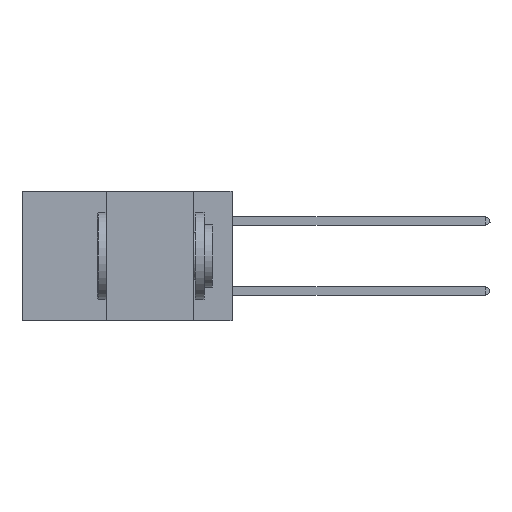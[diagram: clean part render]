
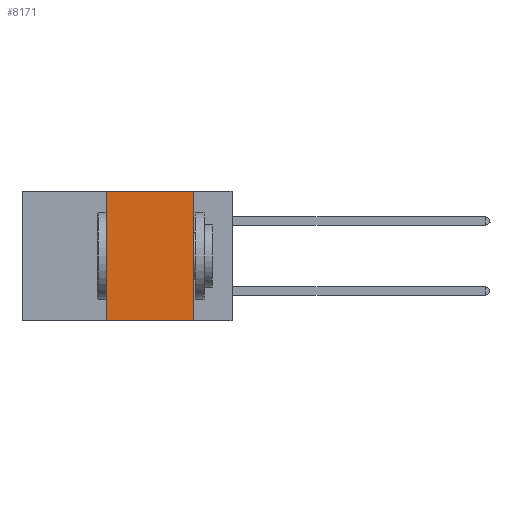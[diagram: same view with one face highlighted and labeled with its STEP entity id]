
A CAD part, left-side view. The second image highlights one B-rep face of the part: STEP entity #8171.
In plain terms, the highlighted planar face has unit normal (-1, 0, 0).
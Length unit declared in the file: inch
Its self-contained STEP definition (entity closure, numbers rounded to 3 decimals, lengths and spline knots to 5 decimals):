
#1097 = CARTESIAN_POINT ( 'NONE',  ( 0., 0.6, -0.37 ) ) ;
#3620 = FACE_OUTER_BOUND ( 'NONE', #18845, .T. ) ;
#3628 = LINE ( 'NONE', #43372, #38370 ) ;
#4054 = ORIENTED_EDGE ( 'NONE', *, *, #33703, .F. ) ;
#4055 = CARTESIAN_POINT ( 'NONE',  ( 0., 0.36, -0.37 ) ) ;
#6452 = DIRECTION ( 'NONE',  ( 0., -1., 0. ) ) ;
#7002 = LINE ( 'NONE', #9540, #31798 ) ;
#7316 = VERTEX_POINT ( 'NONE', #14477 ) ;
#8171 = ADVANCED_FACE ( 'NONE', ( #3620 ), #22578, .F. ) ;
#9113 = CARTESIAN_POINT ( 'NONE',  ( 0., 0.6, 0. ) ) ;
#9540 = CARTESIAN_POINT ( 'NONE',  ( 0., 0.36, 0. ) ) ;
#12536 = DIRECTION ( 'NONE',  ( 0., 0., -1. ) ) ;
#14100 = ORIENTED_EDGE ( 'NONE', *, *, #21582, .T. ) ;
#14477 = CARTESIAN_POINT ( 'NONE',  ( 0., 0.11, 0. ) ) ;
#15210 = CARTESIAN_POINT ( 'NONE',  ( 0., 0.11, 0. ) ) ;
#17832 = EDGE_CURVE ( 'NONE', #7316, #32907, #18195, .T. ) ;
#18195 = LINE ( 'NONE', #15210, #42758 ) ;
#18845 = EDGE_LOOP ( 'NONE', ( #36755, #4054, #39841, #14100 ) ) ;
#19710 = AXIS2_PLACEMENT_3D ( 'NONE', #9113, #32730, #12536 ) ;
#21582 = EDGE_CURVE ( 'NONE', #39195, #32907, #34782, .T. ) ;
#22578 = PLANE ( 'NONE',  #19710 ) ;
#25887 = VECTOR ( 'NONE', #28201, 39.37008 ) ;
#27566 = CARTESIAN_POINT ( 'NONE',  ( 0., 0.36, 0. ) ) ;
#28201 = DIRECTION ( 'NONE',  ( 0., -1., 0. ) ) ;
#29770 = DIRECTION ( 'NONE',  ( 0., 0., 1. ) ) ;
#30534 = EDGE_CURVE ( 'NONE', #39195, #30769, #7002, .T. ) ;
#30769 = VERTEX_POINT ( 'NONE', #27566 ) ;
#31798 = VECTOR ( 'NONE', #29770, 39.37008 ) ;
#32730 = DIRECTION ( 'NONE',  ( 1., 0., 0. ) ) ;
#32907 = VERTEX_POINT ( 'NONE', #38768 ) ;
#33703 = EDGE_CURVE ( 'NONE', #30769, #7316, #3628, .T. ) ;
#34782 = LINE ( 'NONE', #1097, #25887 ) ;
#35351 = DIRECTION ( 'NONE',  ( 0., 0., -1. ) ) ;
#36755 = ORIENTED_EDGE ( 'NONE', *, *, #17832, .F. ) ;
#38370 = VECTOR ( 'NONE', #6452, 39.37008 ) ;
#38768 = CARTESIAN_POINT ( 'NONE',  ( 0., 0.11, -0.37 ) ) ;
#39195 = VERTEX_POINT ( 'NONE', #4055 ) ;
#39841 = ORIENTED_EDGE ( 'NONE', *, *, #30534, .F. ) ;
#42758 = VECTOR ( 'NONE', #35351, 39.37008 ) ;
#43372 = CARTESIAN_POINT ( 'NONE',  ( 0., 0.6, 0. ) ) ;
